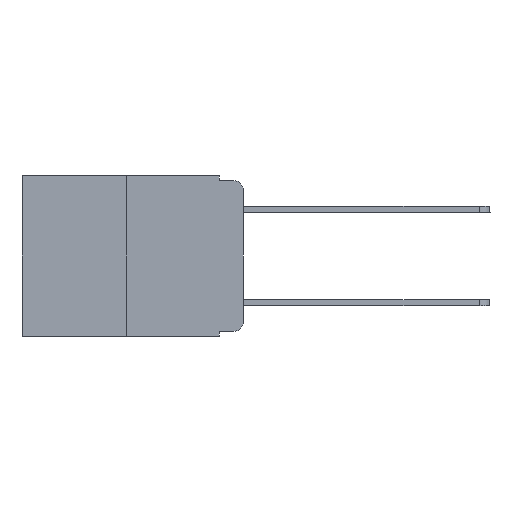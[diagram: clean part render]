
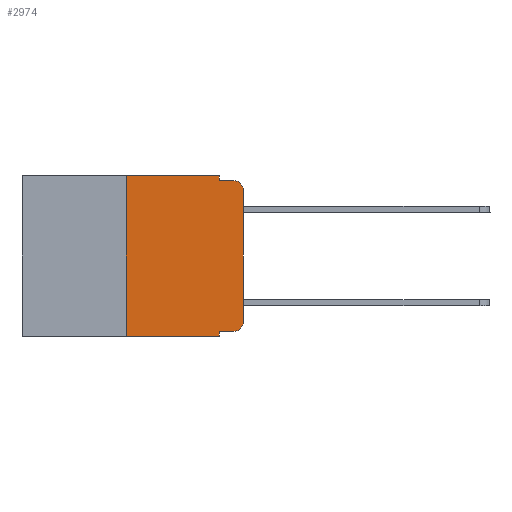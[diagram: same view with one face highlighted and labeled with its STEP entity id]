
A CAD part, left-side view. The second image highlights one B-rep face of the part: STEP entity #2974.
In plain terms, the highlighted planar face has unit normal (-1, 0, 0).
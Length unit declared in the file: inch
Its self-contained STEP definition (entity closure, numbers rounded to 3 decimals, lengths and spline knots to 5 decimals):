
#170 = CARTESIAN_POINT ( 'NONE',  ( 0., 0.25, 0. ) ) ;
#459 = ORIENTED_EDGE ( 'NONE', *, *, #7956, .F. ) ;
#872 = CARTESIAN_POINT ( 'NONE',  ( 0., 0.473, -0.343 ) ) ;
#1151 = DIRECTION ( 'NONE',  ( 0., -1., 0. ) ) ;
#1161 = CARTESIAN_POINT ( 'NONE',  ( 0., 0.051, -0.343 ) ) ;
#1356 = EDGE_CURVE ( 'NONE', #18843, #4280, #12251, .T. ) ;
#2088 = ORIENTED_EDGE ( 'NONE', *, *, #12025, .F. ) ;
#2657 = AXIS2_PLACEMENT_3D ( 'NONE', #3599, #5077, #5313 ) ;
#2974 = ADVANCED_FACE ( 'NONE', ( #10265 ), #4977, .F. ) ;
#3190 = EDGE_CURVE ( 'NONE', #3806, #19568, #8153, .T. ) ;
#3599 = CARTESIAN_POINT ( 'NONE',  ( 0., 0.473, 0. ) ) ;
#3806 = VERTEX_POINT ( 'NONE', #18897 ) ;
#4280 = VERTEX_POINT ( 'NONE', #170 ) ;
#4412 = VERTEX_POINT ( 'NONE', #11325 ) ;
#4977 = PLANE ( 'NONE',  #2657 ) ;
#5077 = DIRECTION ( 'NONE',  ( 1., 0., 0. ) ) ;
#5313 = DIRECTION ( 'NONE',  ( 0., 0., -1. ) ) ;
#5424 = ORIENTED_EDGE ( 'NONE', *, *, #15388, .F. ) ;
#5546 = VECTOR ( 'NONE', #22420, 39.37008 ) ;
#6378 = EDGE_LOOP ( 'NONE', ( #13407, #11359, #21920, #2088, #5424, #14968, #20148, #459, #21854, #13936 ) ) ;
#6460 = DIRECTION ( 'NONE',  ( 0., 0., -1. ) ) ;
#6893 = DIRECTION ( 'NONE',  ( 0., -1., 0. ) ) ;
#6925 = CARTESIAN_POINT ( 'NONE',  ( 0., 0.051, 0. ) ) ;
#6994 = LINE ( 'NONE', #8625, #9317 ) ;
#7127 = DIRECTION ( 'NONE',  ( 0., -1., 0. ) ) ;
#7340 = LINE ( 'NONE', #15885, #8309 ) ;
#7719 = VECTOR ( 'NONE', #8200, 39.37008 ) ;
#7956 = EDGE_CURVE ( 'NONE', #19861, #16963, #10170, .T. ) ;
#8080 = DIRECTION ( 'NONE',  ( 0., -1., 0. ) ) ;
#8153 = CIRCLE ( 'NONE', #14054, 0.02 ) ;
#8200 = DIRECTION ( 'NONE',  ( 0., 0., -1. ) ) ;
#8247 = VERTEX_POINT ( 'NONE', #15339 ) ;
#8252 = VERTEX_POINT ( 'NONE', #20546 ) ;
#8309 = VECTOR ( 'NONE', #7127, 39.37008 ) ;
#8610 = VECTOR ( 'NONE', #20963, 39.37008 ) ;
#8622 = DIRECTION ( 'NONE',  ( -1., 0., 0. ) ) ;
#8625 = CARTESIAN_POINT ( 'NONE',  ( 0., 0.473, 0. ) ) ;
#9317 = VECTOR ( 'NONE', #6893, 39.37008 ) ;
#9561 = CARTESIAN_POINT ( 'NONE',  ( 0., 0.02, -0.313 ) ) ;
#10017 = DIRECTION ( 'NONE',  ( -1., 0., 0. ) ) ;
#10170 = LINE ( 'NONE', #6925, #7719 ) ;
#10255 = LINE ( 'NONE', #12106, #20845 ) ;
#10265 = FACE_OUTER_BOUND ( 'NONE', #6378, .T. ) ;
#10542 = VECTOR ( 'NONE', #1151, 39.37008 ) ;
#11325 = CARTESIAN_POINT ( 'NONE',  ( 0., 0., -0.03 ) ) ;
#11359 = ORIENTED_EDGE ( 'NONE', *, *, #20558, .T. ) ;
#11730 = CARTESIAN_POINT ( 'NONE',  ( 0., 0.051, 0. ) ) ;
#11986 = CARTESIAN_POINT ( 'NONE',  ( 0., 0.02, -0.03 ) ) ;
#12025 = EDGE_CURVE ( 'NONE', #16139, #8247, #18895, .T. ) ;
#12106 = CARTESIAN_POINT ( 'NONE',  ( 0., 0., 0. ) ) ;
#12251 = LINE ( 'NONE', #22326, #5546 ) ;
#12268 = VECTOR ( 'NONE', #8080, 39.37008 ) ;
#13078 = EDGE_CURVE ( 'NONE', #19861, #3806, #7340, .T. ) ;
#13285 = CARTESIAN_POINT ( 'NONE',  ( 0., 0.25, -0.343 ) ) ;
#13407 = ORIENTED_EDGE ( 'NONE', *, *, #18892, .T. ) ;
#13604 = AXIS2_PLACEMENT_3D ( 'NONE', #11986, #8622, #20537 ) ;
#13936 = ORIENTED_EDGE ( 'NONE', *, *, #3190, .T. ) ;
#14054 = AXIS2_PLACEMENT_3D ( 'NONE', #9561, #10017, #6460 ) ;
#14968 = ORIENTED_EDGE ( 'NONE', *, *, #1356, .F. ) ;
#14972 = CARTESIAN_POINT ( 'NONE',  ( 0., 0., -0.313 ) ) ;
#15072 = CARTESIAN_POINT ( 'NONE',  ( 0., 0.051, -0.01 ) ) ;
#15339 = CARTESIAN_POINT ( 'NONE',  ( 0., 0.051, -0.01 ) ) ;
#15388 = EDGE_CURVE ( 'NONE', #4280, #16139, #6994, .T. ) ;
#15852 = CARTESIAN_POINT ( 'NONE',  ( 0., 0.051, -0.333 ) ) ;
#15885 = CARTESIAN_POINT ( 'NONE',  ( 0., 0.051, -0.333 ) ) ;
#16139 = VERTEX_POINT ( 'NONE', #18750 ) ;
#16569 = EDGE_CURVE ( 'NONE', #18843, #16963, #16769, .T. ) ;
#16769 = LINE ( 'NONE', #872, #12268 ) ;
#16963 = VERTEX_POINT ( 'NONE', #1161 ) ;
#17291 = CIRCLE ( 'NONE', #13604, 0.02 ) ;
#18674 = LINE ( 'NONE', #15072, #10542 ) ;
#18750 = CARTESIAN_POINT ( 'NONE',  ( 0., 0.051, 0. ) ) ;
#18843 = VERTEX_POINT ( 'NONE', #13285 ) ;
#18892 = EDGE_CURVE ( 'NONE', #19568, #4412, #10255, .T. ) ;
#18895 = LINE ( 'NONE', #11730, #8610 ) ;
#18897 = CARTESIAN_POINT ( 'NONE',  ( 0., 0.02, -0.333 ) ) ;
#19568 = VERTEX_POINT ( 'NONE', #14972 ) ;
#19755 = EDGE_CURVE ( 'NONE', #8247, #8252, #18674, .T. ) ;
#19861 = VERTEX_POINT ( 'NONE', #15852 ) ;
#20148 = ORIENTED_EDGE ( 'NONE', *, *, #16569, .T. ) ;
#20537 = DIRECTION ( 'NONE',  ( 0., 0., -1. ) ) ;
#20546 = CARTESIAN_POINT ( 'NONE',  ( 0., 0.02, -0.01 ) ) ;
#20558 = EDGE_CURVE ( 'NONE', #4412, #8252, #17291, .T. ) ;
#20845 = VECTOR ( 'NONE', #22296, 39.37008 ) ;
#20963 = DIRECTION ( 'NONE',  ( 0., 0., -1. ) ) ;
#21854 = ORIENTED_EDGE ( 'NONE', *, *, #13078, .T. ) ;
#21920 = ORIENTED_EDGE ( 'NONE', *, *, #19755, .F. ) ;
#22296 = DIRECTION ( 'NONE',  ( 0., 0., 1. ) ) ;
#22326 = CARTESIAN_POINT ( 'NONE',  ( 0., 0.25, 0. ) ) ;
#22420 = DIRECTION ( 'NONE',  ( 0., 0., 1. ) ) ;
